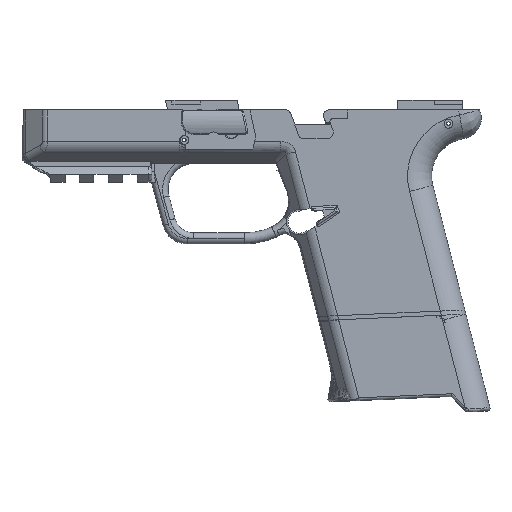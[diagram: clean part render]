
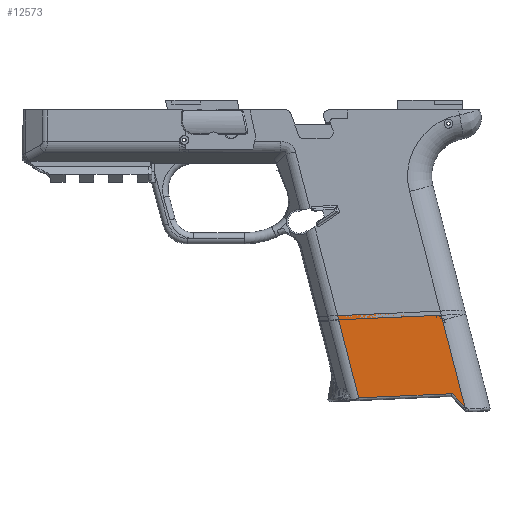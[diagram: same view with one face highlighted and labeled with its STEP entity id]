
A CAD part, left-side view. The second image highlights one B-rep face of the part: STEP entity #12573.
In plain terms, the highlighted face is planar.
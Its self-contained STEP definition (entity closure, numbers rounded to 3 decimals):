
#1044=PLANE('',#13782);
#1720=FACE_OUTER_BOUND('',#2448,.T.);
#2448=EDGE_LOOP('',(#11574,#11575,#11576,#11577,#11578));
#3485=LINE('',#24362,#4566);
#3505=LINE('',#25208,#4586);
#3519=LINE('',#25629,#4600);
#3520=LINE('',#25633,#4601);
#3521=LINE('',#25634,#4602);
#4566=VECTOR('',#16869,10.);
#4586=VECTOR('',#16961,10.);
#4600=VECTOR('',#17033,10.);
#4601=VECTOR('',#17038,10.);
#4602=VECTOR('',#17039,10.);
#6048=VERTEX_POINT('',#24340);
#6050=VERTEX_POINT('',#24360);
#6104=VERTEX_POINT('',#25207);
#6123=VERTEX_POINT('',#25470);
#6131=VERTEX_POINT('',#25632);
#7831=EDGE_CURVE('',#6050,#6048,#3485,.T.);
#7913=EDGE_CURVE('',#6104,#6048,#3505,.T.);
#7958=EDGE_CURVE('',#6123,#6050,#3519,.T.);
#7959=EDGE_CURVE('',#6131,#6123,#3520,.T.);
#7960=EDGE_CURVE('',#6131,#6104,#3521,.T.);
#11574=ORIENTED_EDGE('',*,*,#7831,.F.);
#11575=ORIENTED_EDGE('',*,*,#7958,.F.);
#11576=ORIENTED_EDGE('',*,*,#7959,.F.);
#11577=ORIENTED_EDGE('',*,*,#7960,.T.);
#11578=ORIENTED_EDGE('',*,*,#7913,.T.);
#12573=ADVANCED_FACE('',(#1720),#1044,.T.);
#13782=AXIS2_PLACEMENT_3D('',#25631,#17036,#17037);
#16869=DIRECTION('',(0.,0.999,0.044));
#16961=DIRECTION('',(0.,-0.249,0.969));
#17033=DIRECTION('',(0.,0.697,-0.717));
#17036=DIRECTION('center_axis',(1.,0.,0.));
#17037=DIRECTION('ref_axis',(0.,0.999,0.044));
#17038=DIRECTION('',(0.,-0.249,0.969));
#17039=DIRECTION('',(0.,0.999,0.044));
#24340=CARTESIAN_POINT('',(22.175,-44.727,96.906));
#24360=CARTESIAN_POINT('',(22.175,-78.67,95.402));
#24362=CARTESIAN_POINT('',(22.175,-44.598,96.911));
#25207=CARTESIAN_POINT('',(22.175,-37.062,67.087));
#25208=CARTESIAN_POINT('',(22.175,-37.062,67.087));
#25470=CARTESIAN_POINT('',(22.175,-83.249,100.107));
#25629=CARTESIAN_POINT('',(22.175,-73.025,89.603));
#25631=CARTESIAN_POINT('Origin',(22.175,-74.337,65.435));
#25632=CARTESIAN_POINT('',(22.175,-74.337,65.435));
#25633=CARTESIAN_POINT('',(22.175,-74.337,65.435));
#25634=CARTESIAN_POINT('',(22.175,-40.4,66.939));
